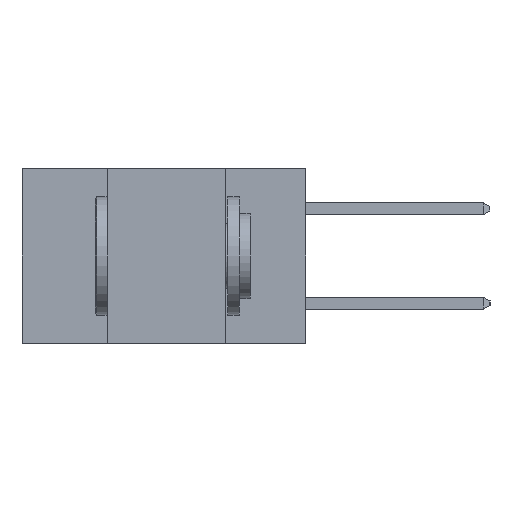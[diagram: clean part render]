
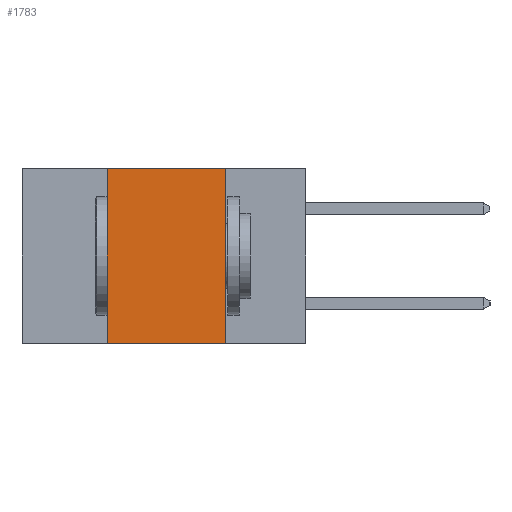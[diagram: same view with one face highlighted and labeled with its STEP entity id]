
A CAD part, left-side view. The second image highlights one B-rep face of the part: STEP entity #1783.
In plain terms, the highlighted planar face has unit normal (-1, 0, 0).
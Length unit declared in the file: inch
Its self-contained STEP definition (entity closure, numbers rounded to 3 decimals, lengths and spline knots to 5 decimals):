
#1496 = EDGE_CURVE ( 'NONE', #19519, #10165, #17442, .T. ) ;
#1783 = ADVANCED_FACE ( 'NONE', ( #12025 ), #8301, .F. ) ;
#2038 = CARTESIAN_POINT ( 'NONE',  ( 0., 0.42, -0.37 ) ) ;
#2867 = DIRECTION ( 'NONE',  ( 0., 0., -1. ) ) ;
#2934 = VECTOR ( 'NONE', #5753, 39.37008 ) ;
#3698 = EDGE_CURVE ( 'NONE', #19519, #10515, #11444, .T. ) ;
#4407 = CARTESIAN_POINT ( 'NONE',  ( 0., 0.6, -0.37 ) ) ;
#5059 = CARTESIAN_POINT ( 'NONE',  ( 0., 0.6, 0. ) ) ;
#5091 = CARTESIAN_POINT ( 'NONE',  ( 0., 0.42, 0. ) ) ;
#5753 = DIRECTION ( 'NONE',  ( 0., -1., 0. ) ) ;
#7362 = DIRECTION ( 'NONE',  ( 0., 0., -1. ) ) ;
#7738 = DIRECTION ( 'NONE',  ( 1., 0., 0. ) ) ;
#7889 = CARTESIAN_POINT ( 'NONE',  ( 0., 0.42, -0.37 ) ) ;
#8031 = CARTESIAN_POINT ( 'NONE',  ( 0., 0.6, 0. ) ) ;
#8301 = PLANE ( 'NONE',  #15924 ) ;
#8755 = DIRECTION ( 'NONE',  ( 0., 0., 1. ) ) ;
#9582 = ORIENTED_EDGE ( 'NONE', *, *, #15536, .F. ) ;
#9783 = ORIENTED_EDGE ( 'NONE', *, *, #19397, .F. ) ;
#9801 = ORIENTED_EDGE ( 'NONE', *, *, #1496, .F. ) ;
#9937 = ORIENTED_EDGE ( 'NONE', *, *, #3698, .T. ) ;
#10165 = VERTEX_POINT ( 'NONE', #5091 ) ;
#10270 = VECTOR ( 'NONE', #2867, 39.37008 ) ;
#10471 = LINE ( 'NONE', #5059, #18862 ) ;
#10494 = VERTEX_POINT ( 'NONE', #15363 ) ;
#10515 = VERTEX_POINT ( 'NONE', #16964 ) ;
#10865 = CARTESIAN_POINT ( 'NONE',  ( 0., 0.17, -0.37 ) ) ;
#11444 = LINE ( 'NONE', #4407, #2934 ) ;
#11742 = EDGE_LOOP ( 'NONE', ( #9582, #9783, #9801, #9937 ) ) ;
#12025 = FACE_OUTER_BOUND ( 'NONE', #11742, .T. ) ;
#14458 = LINE ( 'NONE', #10865, #10270 ) ;
#15363 = CARTESIAN_POINT ( 'NONE',  ( 0., 0.17, 0. ) ) ;
#15536 = EDGE_CURVE ( 'NONE', #10494, #10515, #14458, .T. ) ;
#15924 = AXIS2_PLACEMENT_3D ( 'NONE', #8031, #7738, #7362 ) ;
#16170 = DIRECTION ( 'NONE',  ( 0., -1., 0. ) ) ;
#16964 = CARTESIAN_POINT ( 'NONE',  ( 0., 0.17, -0.37 ) ) ;
#17442 = LINE ( 'NONE', #7889, #20614 ) ;
#18862 = VECTOR ( 'NONE', #16170, 39.37008 ) ;
#19397 = EDGE_CURVE ( 'NONE', #10165, #10494, #10471, .T. ) ;
#19519 = VERTEX_POINT ( 'NONE', #2038 ) ;
#20614 = VECTOR ( 'NONE', #8755, 39.37008 ) ;
